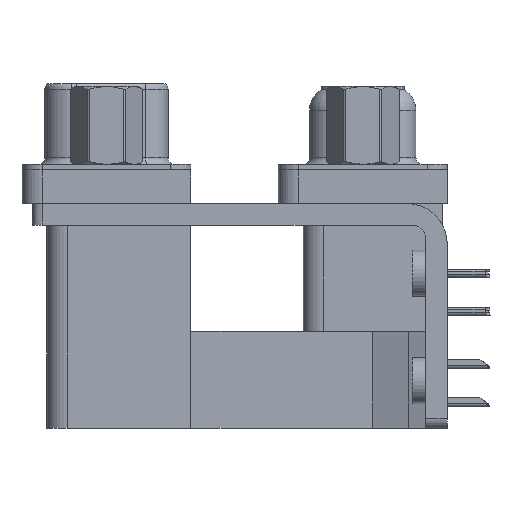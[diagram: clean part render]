
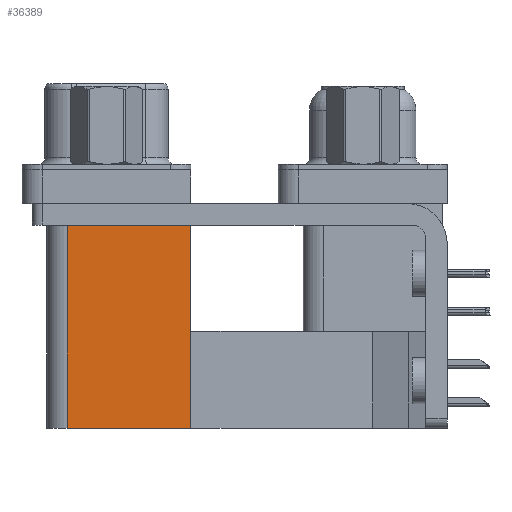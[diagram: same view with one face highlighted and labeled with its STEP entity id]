
A CAD part, left-side view. The second image highlights one B-rep face of the part: STEP entity #36389.
In plain terms, the highlighted planar face has unit normal (-1, 0, 0).
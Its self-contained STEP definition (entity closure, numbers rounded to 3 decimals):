
#2248 = EDGE_CURVE ( 'NONE', #10027, #22056, #40677, .T. ) ;
#4069 = CARTESIAN_POINT ( 'NONE',  ( 3.79, 12.775, -2.5 ) ) ;
#4310 = VECTOR ( 'NONE', #8385, 1000. ) ;
#4356 = AXIS2_PLACEMENT_3D ( 'NONE', #21063, #24001, #34146 ) ;
#5452 = LINE ( 'NONE', #12444, #4310 ) ;
#5693 = ORIENTED_EDGE ( 'NONE', *, *, #23479, .T. ) ;
#5868 = VECTOR ( 'NONE', #16533, 1000. ) ;
#6347 = ORIENTED_EDGE ( 'NONE', *, *, #25600, .F. ) ;
#8385 = DIRECTION ( 'NONE',  ( 0., 0., 1. ) ) ;
#9364 = ORIENTED_EDGE ( 'NONE', *, *, #16313, .T. ) ;
#10027 = VERTEX_POINT ( 'NONE', #31285 ) ;
#12444 = CARTESIAN_POINT ( 'NONE',  ( 3.79, 12.775, -19.2 ) ) ;
#15704 = CARTESIAN_POINT ( 'NONE',  ( 3.79, 12.775, -19.2 ) ) ;
#16134 = CARTESIAN_POINT ( 'NONE',  ( 3.79, 21.975, -19.2 ) ) ;
#16313 = EDGE_CURVE ( 'NONE', #39218, #23245, #5452, .T. ) ;
#16533 = DIRECTION ( 'NONE',  ( 0., 1., 0. ) ) ;
#16672 = LINE ( 'NONE', #36759, #43166 ) ;
#17667 = PLANE ( 'NONE',  #4356 ) ;
#21063 = CARTESIAN_POINT ( 'NONE',  ( 3.79, 12.775, -19.2 ) ) ;
#21437 = CARTESIAN_POINT ( 'NONE',  ( 3.79, 12.775, -19.2 ) ) ;
#22056 = VERTEX_POINT ( 'NONE', #32555 ) ;
#22677 = FACE_OUTER_BOUND ( 'NONE', #28607, .T. ) ;
#23245 = VERTEX_POINT ( 'NONE', #4069 ) ;
#23479 = EDGE_CURVE ( 'NONE', #23245, #22056, #16672, .T. ) ;
#24001 = DIRECTION ( 'NONE',  ( 1., 0., 0. ) ) ;
#25600 = EDGE_CURVE ( 'NONE', #39218, #10027, #33906, .T. ) ;
#28607 = EDGE_LOOP ( 'NONE', ( #5693, #39926, #6347, #9364 ) ) ;
#31285 = CARTESIAN_POINT ( 'NONE',  ( 3.79, 21.975, -19.2 ) ) ;
#32555 = CARTESIAN_POINT ( 'NONE',  ( 3.79, 21.975, -2.5 ) ) ;
#33169 = DIRECTION ( 'NONE',  ( 0., 1., 0. ) ) ;
#33906 = LINE ( 'NONE', #15704, #5868 ) ;
#34146 = DIRECTION ( 'NONE',  ( 0., 0., -1. ) ) ;
#34208 = VECTOR ( 'NONE', #37304, 1000. ) ;
#36389 = ADVANCED_FACE ( 'NONE', ( #22677 ), #17667, .F. ) ;
#36759 = CARTESIAN_POINT ( 'NONE',  ( 3.79, 12.775, -2.5 ) ) ;
#37304 = DIRECTION ( 'NONE',  ( 0., 0., 1. ) ) ;
#39218 = VERTEX_POINT ( 'NONE', #21437 ) ;
#39926 = ORIENTED_EDGE ( 'NONE', *, *, #2248, .F. ) ;
#40677 = LINE ( 'NONE', #16134, #34208 ) ;
#43166 = VECTOR ( 'NONE', #33169, 1000. ) ;
